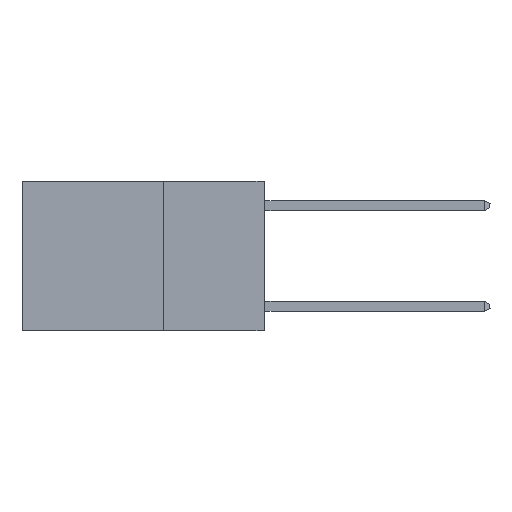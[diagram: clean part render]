
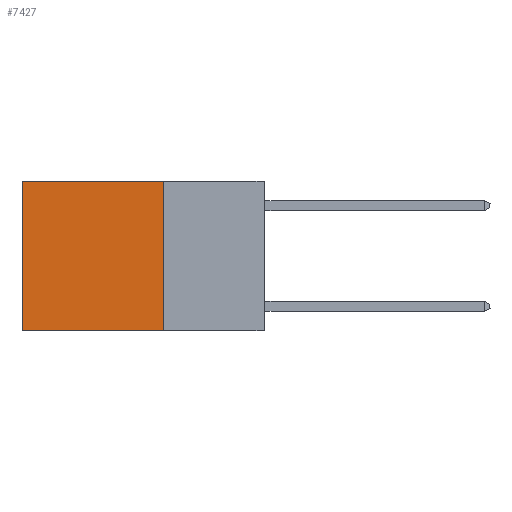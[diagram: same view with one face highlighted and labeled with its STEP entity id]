
A CAD part, left-side view. The second image highlights one B-rep face of the part: STEP entity #7427.
In plain terms, the highlighted planar face has unit normal (-1, 0, 0).
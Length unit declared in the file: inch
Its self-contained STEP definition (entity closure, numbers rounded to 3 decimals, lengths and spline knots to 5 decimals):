
#92 = CARTESIAN_POINT ( 'NONE',  ( 0.2625, 0.6, 0. ) ) ;
#564 = DIRECTION ( 'NONE',  ( 0., 0., -1. ) ) ;
#965 = AXIS2_PLACEMENT_3D ( 'NONE', #6279, #3541, #2861 ) ;
#1644 = LINE ( 'NONE', #7515, #9013 ) ;
#2102 = CARTESIAN_POINT ( 'NONE',  ( 0.2625, 0.25, -0.37 ) ) ;
#2861 = DIRECTION ( 'NONE',  ( 0., 0., -1. ) ) ;
#3255 = PLANE ( 'NONE',  #965 ) ;
#3310 = ORIENTED_EDGE ( 'NONE', *, *, #8342, .F. ) ;
#3541 = DIRECTION ( 'NONE',  ( 1., 0., 0. ) ) ;
#4038 = VECTOR ( 'NONE', #9069, 39.37008 ) ;
#4388 = ORIENTED_EDGE ( 'NONE', *, *, #5159, .T. ) ;
#4401 = VERTEX_POINT ( 'NONE', #92 ) ;
#4529 = EDGE_CURVE ( 'NONE', #9488, #4401, #9802, .T. ) ;
#4570 = CARTESIAN_POINT ( 'NONE',  ( 0.2625, 0.25, 0. ) ) ;
#4915 = LINE ( 'NONE', #8397, #9938 ) ;
#5159 = EDGE_CURVE ( 'NONE', #4401, #7363, #4915, .T. ) ;
#5345 = DIRECTION ( 'NONE',  ( 0., 1., 0. ) ) ;
#5833 = EDGE_CURVE ( 'NONE', #11070, #7363, #9749, .T. ) ;
#5885 = CARTESIAN_POINT ( 'NONE',  ( 0.2625, 0.6, -0.37 ) ) ;
#6279 = CARTESIAN_POINT ( 'NONE',  ( 0.2625, 0.25, 0. ) ) ;
#6571 = ORIENTED_EDGE ( 'NONE', *, *, #4529, .T. ) ;
#7350 = CARTESIAN_POINT ( 'NONE',  ( 0.2625, 0.25, -0.37 ) ) ;
#7363 = VERTEX_POINT ( 'NONE', #5885 ) ;
#7427 = ADVANCED_FACE ( 'NONE', ( #8459 ), #3255, .F. ) ;
#7515 = CARTESIAN_POINT ( 'NONE',  ( 0.2625, 0.25, 0. ) ) ;
#7619 = ORIENTED_EDGE ( 'NONE', *, *, #5833, .F. ) ;
#7790 = EDGE_LOOP ( 'NONE', ( #4388, #7619, #3310, #6571 ) ) ;
#8342 = EDGE_CURVE ( 'NONE', #9488, #11070, #1644, .T. ) ;
#8397 = CARTESIAN_POINT ( 'NONE',  ( 0.2625, 0.6, 0. ) ) ;
#8459 = FACE_OUTER_BOUND ( 'NONE', #7790, .T. ) ;
#8685 = VECTOR ( 'NONE', #5345, 39.37008 ) ;
#9013 = VECTOR ( 'NONE', #11101, 39.37008 ) ;
#9069 = DIRECTION ( 'NONE',  ( 0., 1., 0. ) ) ;
#9488 = VERTEX_POINT ( 'NONE', #9861 ) ;
#9749 = LINE ( 'NONE', #2102, #4038 ) ;
#9802 = LINE ( 'NONE', #4570, #8685 ) ;
#9861 = CARTESIAN_POINT ( 'NONE',  ( 0.2625, 0.25, 0. ) ) ;
#9938 = VECTOR ( 'NONE', #564, 39.37008 ) ;
#11070 = VERTEX_POINT ( 'NONE', #7350 ) ;
#11101 = DIRECTION ( 'NONE',  ( 0., 0., -1. ) ) ;
